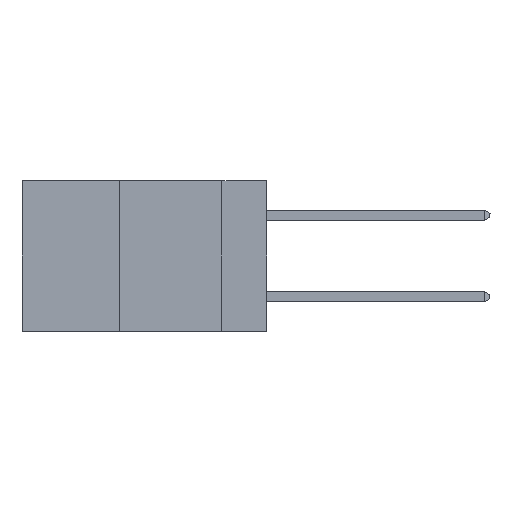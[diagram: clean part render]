
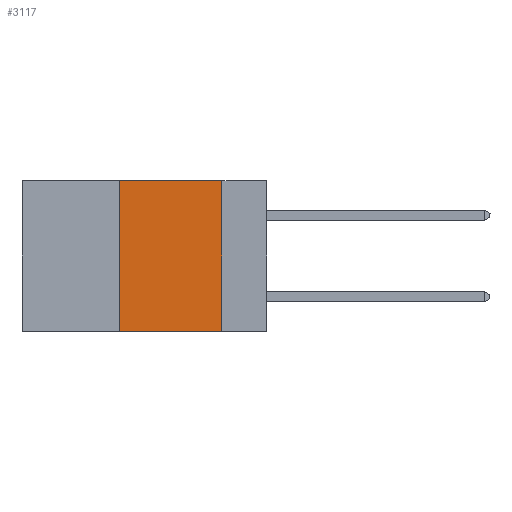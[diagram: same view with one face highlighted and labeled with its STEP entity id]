
A CAD part, left-side view. The second image highlights one B-rep face of the part: STEP entity #3117.
In plain terms, the highlighted planar face has unit normal (-1, 0, 0).
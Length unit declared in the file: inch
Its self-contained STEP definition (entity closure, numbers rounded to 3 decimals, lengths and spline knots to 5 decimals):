
#716 = CARTESIAN_POINT ( 'NONE',  ( 0., 0.6, -0.37 ) ) ;
#868 = ORIENTED_EDGE ( 'NONE', *, *, #15157, .F. ) ;
#1204 = DIRECTION ( 'NONE',  ( 0., 0., -1. ) ) ;
#2208 = CARTESIAN_POINT ( 'NONE',  ( 0., 0.11, 0. ) ) ;
#2272 = VECTOR ( 'NONE', #7117, 39.37008 ) ;
#2358 = EDGE_CURVE ( 'NONE', #14108, #13186, #6671, .T. ) ;
#3117 = ADVANCED_FACE ( 'NONE', ( #17018 ), #15721, .F. ) ;
#3755 = DIRECTION ( 'NONE',  ( 1., 0., 0. ) ) ;
#4311 = LINE ( 'NONE', #7018, #2272 ) ;
#4408 = CARTESIAN_POINT ( 'NONE',  ( 0., 0.6, 0. ) ) ;
#4528 = VECTOR ( 'NONE', #14071, 39.37008 ) ;
#4928 = LINE ( 'NONE', #716, #17275 ) ;
#6172 = VERTEX_POINT ( 'NONE', #11597 ) ;
#6671 = LINE ( 'NONE', #4408, #13792 ) ;
#6796 = ORIENTED_EDGE ( 'NONE', *, *, #2358, .F. ) ;
#7018 = CARTESIAN_POINT ( 'NONE',  ( 0., 0.36, 0. ) ) ;
#7034 = DIRECTION ( 'NONE',  ( 0., -1., 0. ) ) ;
#7117 = DIRECTION ( 'NONE',  ( 0., 0., 1. ) ) ;
#7892 = VERTEX_POINT ( 'NONE', #10023 ) ;
#8760 = LINE ( 'NONE', #2208, #4528 ) ;
#9787 = ORIENTED_EDGE ( 'NONE', *, *, #17241, .F. ) ;
#10023 = CARTESIAN_POINT ( 'NONE',  ( 0., 0.11, -0.37 ) ) ;
#10208 = CARTESIAN_POINT ( 'NONE',  ( 0., 0.6, 0. ) ) ;
#10385 = CARTESIAN_POINT ( 'NONE',  ( 0., 0.11, 0. ) ) ;
#10406 = CARTESIAN_POINT ( 'NONE',  ( 0., 0.36, 0. ) ) ;
#11597 = CARTESIAN_POINT ( 'NONE',  ( 0., 0.36, -0.37 ) ) ;
#11609 = DIRECTION ( 'NONE',  ( 0., -1., 0. ) ) ;
#11860 = AXIS2_PLACEMENT_3D ( 'NONE', #10208, #3755, #1204 ) ;
#13056 = EDGE_LOOP ( 'NONE', ( #868, #6796, #9787, #14586 ) ) ;
#13178 = EDGE_CURVE ( 'NONE', #6172, #7892, #4928, .T. ) ;
#13186 = VERTEX_POINT ( 'NONE', #10385 ) ;
#13792 = VECTOR ( 'NONE', #7034, 39.37008 ) ;
#14071 = DIRECTION ( 'NONE',  ( 0., 0., -1. ) ) ;
#14108 = VERTEX_POINT ( 'NONE', #10406 ) ;
#14586 = ORIENTED_EDGE ( 'NONE', *, *, #13178, .T. ) ;
#15157 = EDGE_CURVE ( 'NONE', #13186, #7892, #8760, .T. ) ;
#15721 = PLANE ( 'NONE',  #11860 ) ;
#17018 = FACE_OUTER_BOUND ( 'NONE', #13056, .T. ) ;
#17241 = EDGE_CURVE ( 'NONE', #6172, #14108, #4311, .T. ) ;
#17275 = VECTOR ( 'NONE', #11609, 39.37008 ) ;
